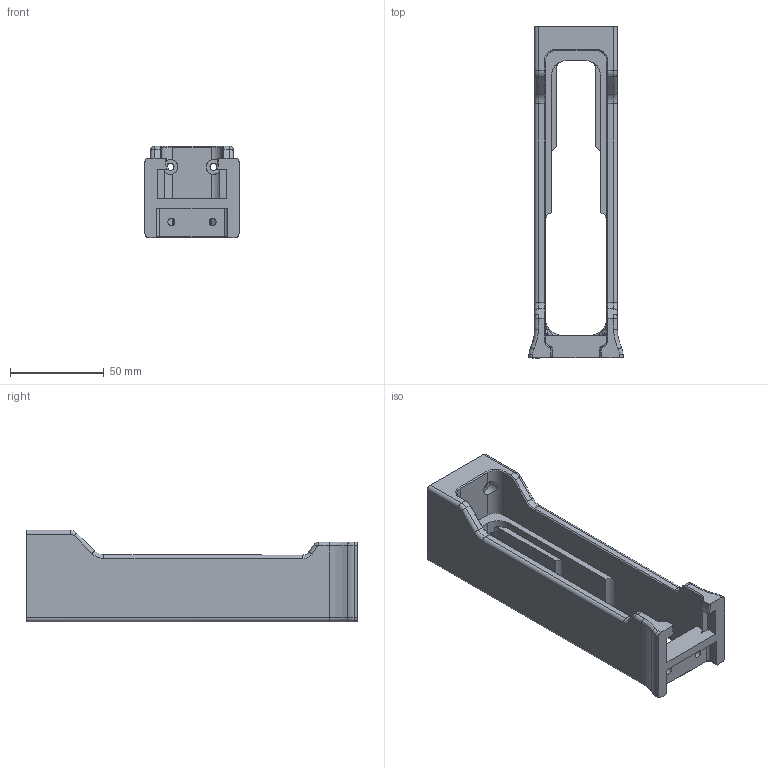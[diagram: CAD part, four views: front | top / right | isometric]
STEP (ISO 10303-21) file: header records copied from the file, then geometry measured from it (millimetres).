
FILE_DESCRIPTION(/* description */ (''),/* implementation_level */ '2;1');
FILE_NAME(/* name */ 'Mid Chassis.step',/* time_stamp */ '2021-08-06T21:52:29-04:00',/* author */ (''),/* organization */ (''),/* preprocessor_version */ 'ST-DEVELOPER v18.1',/* originating_system */ 'Autodesk Translation Framework v10.9.0.1377',/* authorisation */ '');
FILE_SCHEMA (('AUTOMOTIVE_DESIGN { 1 0 10303 214 3 1 1 }'));
Length unit declared in the file: millimetre
Products named in the file (1): Mid Chassis
Bounding box: 50.15 x 177 x 48.8 mm (x, y, z)
Volume: 117742.3 mm3; surface area: 39862.2 mm2
Topology: 1 solids, 1 shells, 267 faces, 683 edges, 412 vertices
Faces by surface type: plane 103, cylinder 74, bspline 44, cone 24, torus 20, sphere 2
Full cylindrical faces by diameter (mm): 3.8 x4, 8 x4
Entity records: 9458 total; most frequent: CARTESIAN_POINT 3175, ORIENTED_EDGE 1358, DIRECTION 1241, EDGE_CURVE 679, AXIS2_PLACEMENT_3D 449, VERTEX_POINT 412, LINE 343, VECTOR 343
